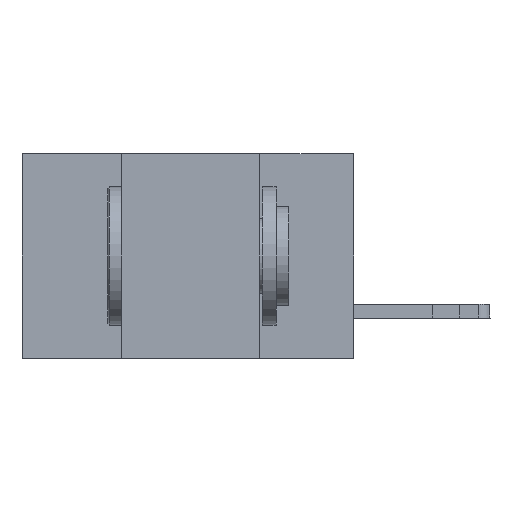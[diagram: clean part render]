
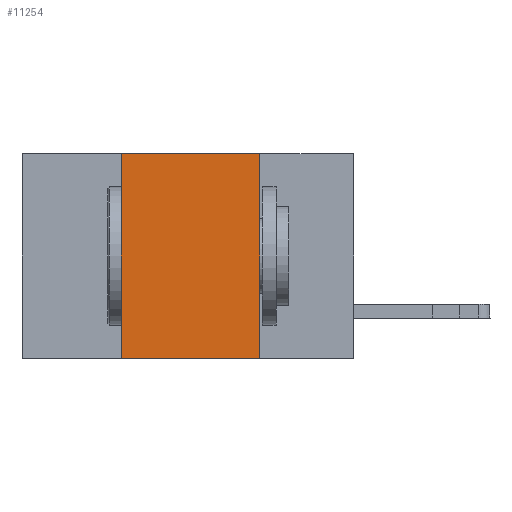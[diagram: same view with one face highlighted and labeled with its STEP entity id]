
A CAD part, left-side view. The second image highlights one B-rep face of the part: STEP entity #11254.
In plain terms, the highlighted planar face has unit normal (-1, 0, 0).
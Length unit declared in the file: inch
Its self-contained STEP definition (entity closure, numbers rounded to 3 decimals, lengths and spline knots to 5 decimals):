
#806 = VECTOR ( 'NONE', #14117, 39.37008 ) ;
#996 = DIRECTION ( 'NONE',  ( 0., 0., -1. ) ) ;
#2035 = ORIENTED_EDGE ( 'NONE', *, *, #3539, .F. ) ;
#2056 = CARTESIAN_POINT ( 'NONE',  ( 0., 0.6, 0. ) ) ;
#2830 = CARTESIAN_POINT ( 'NONE',  ( 0., 0.17, 0. ) ) ;
#3511 = LINE ( 'NONE', #3919, #14714 ) ;
#3539 = EDGE_CURVE ( 'NONE', #6434, #14145, #19502, .T. ) ;
#3596 = ORIENTED_EDGE ( 'NONE', *, *, #28456, .F. ) ;
#3778 = ORIENTED_EDGE ( 'NONE', *, *, #8951, .F. ) ;
#3919 = CARTESIAN_POINT ( 'NONE',  ( 0., 0.42, 0. ) ) ;
#4412 = CARTESIAN_POINT ( 'NONE',  ( 0., 0.6, -0.37 ) ) ;
#5462 = ORIENTED_EDGE ( 'NONE', *, *, #14849, .T. ) ;
#6197 = DIRECTION ( 'NONE',  ( 0., 0., 1. ) ) ;
#6434 = VERTEX_POINT ( 'NONE', #21568 ) ;
#6689 = DIRECTION ( 'NONE',  ( 0., -1., 0. ) ) ;
#6884 = LINE ( 'NONE', #2830, #806 ) ;
#7054 = FACE_OUTER_BOUND ( 'NONE', #20915, .T. ) ;
#7789 = CARTESIAN_POINT ( 'NONE',  ( 0., 0.6, 0. ) ) ;
#8951 = EDGE_CURVE ( 'NONE', #16838, #6434, #3511, .T. ) ;
#10434 = CARTESIAN_POINT ( 'NONE',  ( 0., 0.17, 0. ) ) ;
#11254 = ADVANCED_FACE ( 'NONE', ( #7054 ), #27436, .F. ) ;
#12274 = VECTOR ( 'NONE', #28441, 39.37008 ) ;
#13513 = AXIS2_PLACEMENT_3D ( 'NONE', #7789, #14470, #996 ) ;
#14117 = DIRECTION ( 'NONE',  ( 0., 0., -1. ) ) ;
#14145 = VERTEX_POINT ( 'NONE', #10434 ) ;
#14470 = DIRECTION ( 'NONE',  ( 1., 0., 0. ) ) ;
#14714 = VECTOR ( 'NONE', #6197, 39.37008 ) ;
#14849 = EDGE_CURVE ( 'NONE', #16838, #23765, #25681, .T. ) ;
#16838 = VERTEX_POINT ( 'NONE', #23328 ) ;
#16997 = CARTESIAN_POINT ( 'NONE',  ( 0., 0.17, -0.37 ) ) ;
#19502 = LINE ( 'NONE', #2056, #12274 ) ;
#20915 = EDGE_LOOP ( 'NONE', ( #3596, #2035, #3778, #5462 ) ) ;
#21568 = CARTESIAN_POINT ( 'NONE',  ( 0., 0.42, 0. ) ) ;
#23328 = CARTESIAN_POINT ( 'NONE',  ( 0., 0.42, -0.37 ) ) ;
#23765 = VERTEX_POINT ( 'NONE', #16997 ) ;
#25021 = VECTOR ( 'NONE', #6689, 39.37008 ) ;
#25681 = LINE ( 'NONE', #4412, #25021 ) ;
#27436 = PLANE ( 'NONE',  #13513 ) ;
#28441 = DIRECTION ( 'NONE',  ( 0., -1., 0. ) ) ;
#28456 = EDGE_CURVE ( 'NONE', #14145, #23765, #6884, .T. ) ;
